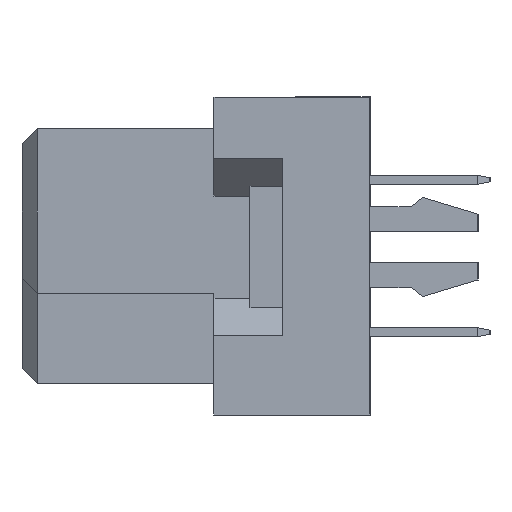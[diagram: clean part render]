
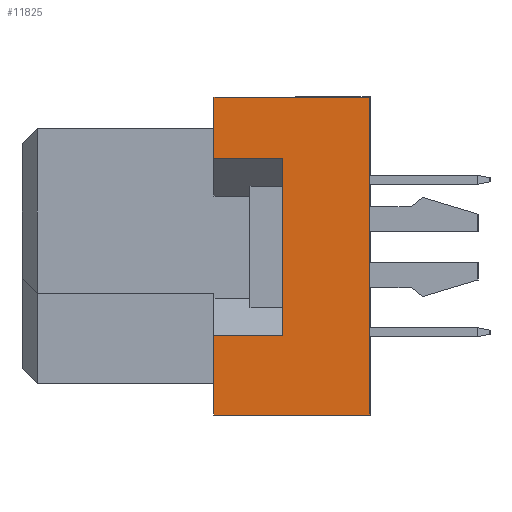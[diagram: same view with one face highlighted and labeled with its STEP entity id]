
A CAD part, left-side view. The second image highlights one B-rep face of the part: STEP entity #11825.
In plain terms, the highlighted planar face has unit normal (-1, 0, 0).
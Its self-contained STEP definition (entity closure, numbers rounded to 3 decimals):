
#426 = LINE ( 'NONE', #24338, #24894 ) ;
#735 = DIRECTION ( 'NONE',  ( 0., 1., 0. ) ) ;
#741 = CARTESIAN_POINT ( 'NONE',  ( -47.5, -8.7, -2.65 ) ) ;
#1526 = EDGE_CURVE ( 'NONE', #5426, #5498, #36176, .T. ) ;
#3707 = CARTESIAN_POINT ( 'NONE',  ( -47.5, -6.4, -2.65 ) ) ;
#4978 = ORIENTED_EDGE ( 'NONE', *, *, #35966, .F. ) ;
#5032 = EDGE_CURVE ( 'NONE', #11839, #15655, #29452, .T. ) ;
#5426 = VERTEX_POINT ( 'NONE', #8221 ) ;
#5498 = VERTEX_POINT ( 'NONE', #12196 ) ;
#7669 = AXIS2_PLACEMENT_3D ( 'NONE', #30607, #21436, #30816 ) ;
#7839 = CARTESIAN_POINT ( 'NONE',  ( -47.5, -6.4, -5.3 ) ) ;
#7873 = EDGE_CURVE ( 'NONE', #33437, #15655, #22091, .T. ) ;
#8221 = CARTESIAN_POINT ( 'NONE',  ( -47.5, -8.7, 3.25 ) ) ;
#8310 = DIRECTION ( 'NONE',  ( 0., 0., 1. ) ) ;
#9404 = DIRECTION ( 'NONE',  ( 0., 0., 1. ) ) ;
#9670 = PLANE ( 'NONE',  #7669 ) ;
#9937 = VECTOR ( 'NONE', #27003, 1000. ) ;
#10114 = CARTESIAN_POINT ( 'NONE',  ( -47.5, -11.6, 5.3 ) ) ;
#10212 = ORIENTED_EDGE ( 'NONE', *, *, #10268, .F. ) ;
#10268 = EDGE_CURVE ( 'NONE', #33437, #5426, #426, .T. ) ;
#11381 = EDGE_CURVE ( 'NONE', #15914, #39068, #33647, .T. ) ;
#11825 = ADVANCED_FACE ( 'NONE', ( #36982 ), #9670, .T. ) ;
#11839 = VERTEX_POINT ( 'NONE', #25793 ) ;
#12196 = CARTESIAN_POINT ( 'NONE',  ( -47.5, -6.4, 3.25 ) ) ;
#14031 = LINE ( 'NONE', #7839, #38929 ) ;
#14267 = CARTESIAN_POINT ( 'NONE',  ( -47.5, -11.6, -5.3 ) ) ;
#14561 = ORIENTED_EDGE ( 'NONE', *, *, #33270, .T. ) ;
#15380 = VERTEX_POINT ( 'NONE', #34499 ) ;
#15655 = VERTEX_POINT ( 'NONE', #3707 ) ;
#15914 = VERTEX_POINT ( 'NONE', #29794 ) ;
#17167 = LINE ( 'NONE', #35107, #17794 ) ;
#17794 = VECTOR ( 'NONE', #35507, 1000. ) ;
#17828 = CARTESIAN_POINT ( 'NONE',  ( -47.5, -8.7, 3.25 ) ) ;
#18306 = DIRECTION ( 'NONE',  ( 0., 1., 0. ) ) ;
#21117 = VECTOR ( 'NONE', #18306, 1000. ) ;
#21436 = DIRECTION ( 'NONE',  ( -1., 0., 0. ) ) ;
#22091 = LINE ( 'NONE', #741, #21117 ) ;
#22923 = VECTOR ( 'NONE', #735, 1000. ) ;
#23776 = VECTOR ( 'NONE', #29402, 1000. ) ;
#24023 = ORIENTED_EDGE ( 'NONE', *, *, #1526, .F. ) ;
#24112 = CARTESIAN_POINT ( 'NONE',  ( -47.5, -8.7, -2.65 ) ) ;
#24338 = CARTESIAN_POINT ( 'NONE',  ( -47.5, -8.7, -2.65 ) ) ;
#24769 = ORIENTED_EDGE ( 'NONE', *, *, #5032, .F. ) ;
#24894 = VECTOR ( 'NONE', #9404, 1000. ) ;
#25504 = CARTESIAN_POINT ( 'NONE',  ( -47.5, -6.4, 5.3 ) ) ;
#25793 = CARTESIAN_POINT ( 'NONE',  ( -47.5, -6.4, -5.3 ) ) ;
#27003 = DIRECTION ( 'NONE',  ( 0., 1., 0. ) ) ;
#28213 = ORIENTED_EDGE ( 'NONE', *, *, #11381, .T. ) ;
#29326 = EDGE_CURVE ( 'NONE', #15380, #11839, #35578, .T. ) ;
#29402 = DIRECTION ( 'NONE',  ( 0., 1., 0. ) ) ;
#29452 = LINE ( 'NONE', #35627, #31161 ) ;
#29794 = CARTESIAN_POINT ( 'NONE',  ( -47.5, -11.6, 5.3 ) ) ;
#30607 = CARTESIAN_POINT ( 'NONE',  ( -47.5, -11.6, 5.3 ) ) ;
#30816 = DIRECTION ( 'NONE',  ( 0., 0., 1. ) ) ;
#31161 = VECTOR ( 'NONE', #8310, 1000. ) ;
#33270 = EDGE_CURVE ( 'NONE', #15380, #15914, #17167, .T. ) ;
#33437 = VERTEX_POINT ( 'NONE', #24112 ) ;
#33647 = LINE ( 'NONE', #10114, #22923 ) ;
#34499 = CARTESIAN_POINT ( 'NONE',  ( -47.5, -11.6, -5.3 ) ) ;
#35011 = ORIENTED_EDGE ( 'NONE', *, *, #29326, .F. ) ;
#35107 = CARTESIAN_POINT ( 'NONE',  ( -47.5, -11.6, 5.3 ) ) ;
#35507 = DIRECTION ( 'NONE',  ( 0., 0., 1. ) ) ;
#35578 = LINE ( 'NONE', #14267, #23776 ) ;
#35627 = CARTESIAN_POINT ( 'NONE',  ( -47.5, -6.4, -5.3 ) ) ;
#35966 = EDGE_CURVE ( 'NONE', #5498, #39068, #14031, .T. ) ;
#36176 = LINE ( 'NONE', #17828, #9937 ) ;
#36982 = FACE_OUTER_BOUND ( 'NONE', #38679, .T. ) ;
#37533 = ORIENTED_EDGE ( 'NONE', *, *, #7873, .T. ) ;
#38146 = DIRECTION ( 'NONE',  ( 0., 0., 1. ) ) ;
#38679 = EDGE_LOOP ( 'NONE', ( #37533, #24769, #35011, #14561, #28213, #4978, #24023, #10212 ) ) ;
#38929 = VECTOR ( 'NONE', #38146, 1000. ) ;
#39068 = VERTEX_POINT ( 'NONE', #25504 ) ;
